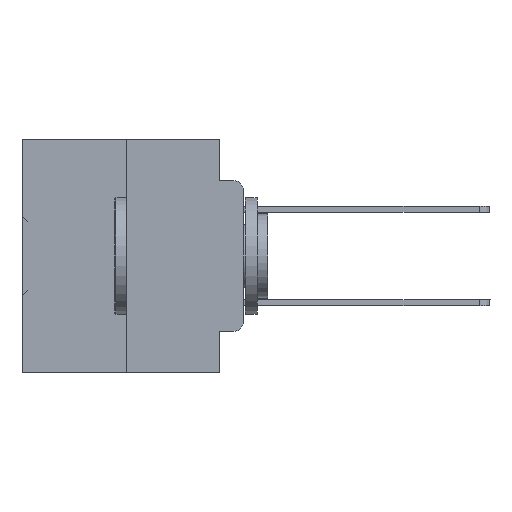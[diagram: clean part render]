
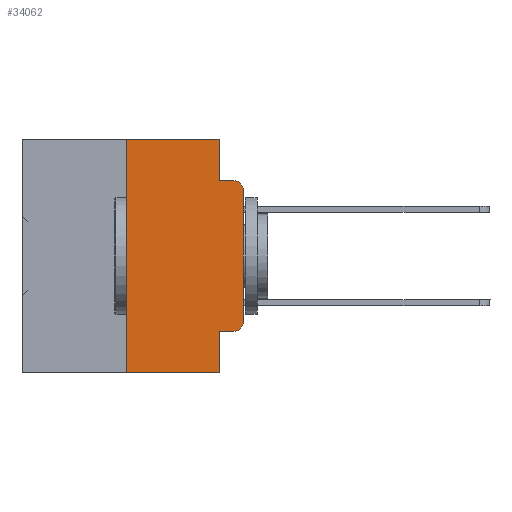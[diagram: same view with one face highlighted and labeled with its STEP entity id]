
A CAD part, left-side view. The second image highlights one B-rep face of the part: STEP entity #34062.
In plain terms, the highlighted planar face has unit normal (-1, 0, 0).
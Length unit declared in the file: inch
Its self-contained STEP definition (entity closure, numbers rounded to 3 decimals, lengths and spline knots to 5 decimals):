
#407 = VERTEX_POINT ( 'NONE', #38082 ) ;
#683 = VECTOR ( 'NONE', #4241, 39.37008 ) ;
#1294 = VERTEX_POINT ( 'NONE', #4804 ) ;
#1327 = CARTESIAN_POINT ( 'NONE',  ( 0., 0.02, -0.1085 ) ) ;
#2591 = VERTEX_POINT ( 'NONE', #18202 ) ;
#2975 = AXIS2_PLACEMENT_3D ( 'NONE', #17209, #35795, #11533 ) ;
#3467 = DIRECTION ( 'NONE',  ( 0., 0., 1. ) ) ;
#3710 = CARTESIAN_POINT ( 'NONE',  ( 0., 0.25, -0.5 ) ) ;
#3954 = VECTOR ( 'NONE', #31752, 39.37008 ) ;
#4241 = DIRECTION ( 'NONE',  ( 0., 0., 1. ) ) ;
#4332 = DIRECTION ( 'NONE',  ( 0., 0., -1. ) ) ;
#4364 = ORIENTED_EDGE ( 'NONE', *, *, #11351, .T. ) ;
#4804 = CARTESIAN_POINT ( 'NONE',  ( 0., 0.25, 0. ) ) ;
#6156 = DIRECTION ( 'NONE',  ( 0., -1., 0. ) ) ;
#6776 = DIRECTION ( 'NONE',  ( 0., 0., -1. ) ) ;
#6973 = DIRECTION ( 'NONE',  ( -1., 0., 0. ) ) ;
#7089 = VERTEX_POINT ( 'NONE', #38326 ) ;
#7437 = VERTEX_POINT ( 'NONE', #3710 ) ;
#8214 = VERTEX_POINT ( 'NONE', #8440 ) ;
#8440 = CARTESIAN_POINT ( 'NONE',  ( 0., 0.051, -0.5 ) ) ;
#8843 = VECTOR ( 'NONE', #4332, 39.37008 ) ;
#9955 = EDGE_CURVE ( 'NONE', #7089, #17361, #34268, .T. ) ;
#10130 = VERTEX_POINT ( 'NONE', #12639 ) ;
#11351 = EDGE_CURVE ( 'NONE', #17361, #12760, #29073, .T. ) ;
#11533 = DIRECTION ( 'NONE',  ( 0., 0., -1. ) ) ;
#11963 = EDGE_CURVE ( 'NONE', #2591, #26058, #12792, .T. ) ;
#12149 = CARTESIAN_POINT ( 'NONE',  ( 0., 0.25, 0. ) ) ;
#12639 = CARTESIAN_POINT ( 'NONE',  ( 0., 0.051, -0.4115 ) ) ;
#12760 = VERTEX_POINT ( 'NONE', #35801 ) ;
#12792 = LINE ( 'NONE', #28317, #3954 ) ;
#12915 = LINE ( 'NONE', #34125, #22692 ) ;
#13375 = LINE ( 'NONE', #31732, #28766 ) ;
#13603 = CIRCLE ( 'NONE', #23914, 0.02 ) ;
#14032 = LINE ( 'NONE', #31983, #8843 ) ;
#14511 = LINE ( 'NONE', #17930, #18230 ) ;
#15934 = EDGE_CURVE ( 'NONE', #7437, #1294, #37210, .T. ) ;
#17081 = EDGE_CURVE ( 'NONE', #12760, #26058, #13603, .T. ) ;
#17209 = CARTESIAN_POINT ( 'NONE',  ( 0., 0.473, 0. ) ) ;
#17314 = DIRECTION ( 'NONE',  ( 0., 0., -1. ) ) ;
#17361 = VERTEX_POINT ( 'NONE', #30176 ) ;
#17407 = VECTOR ( 'NONE', #3467, 39.37008 ) ;
#17795 = FACE_OUTER_BOUND ( 'NONE', #28862, .T. ) ;
#17930 = CARTESIAN_POINT ( 'NONE',  ( 0., 0.051, 0. ) ) ;
#18202 = CARTESIAN_POINT ( 'NONE',  ( 0., 0.051, -0.0885 ) ) ;
#18230 = VECTOR ( 'NONE', #26824, 39.37008 ) ;
#18238 = ORIENTED_EDGE ( 'NONE', *, *, #34760, .F. ) ;
#18348 = ORIENTED_EDGE ( 'NONE', *, *, #9955, .T. ) ;
#18713 = EDGE_CURVE ( 'NONE', #407, #2591, #14511, .T. ) ;
#19582 = EDGE_CURVE ( 'NONE', #1294, #407, #12915, .T. ) ;
#19588 = ORIENTED_EDGE ( 'NONE', *, *, #15934, .F. ) ;
#20094 = AXIS2_PLACEMENT_3D ( 'NONE', #33239, #32841, #17314 ) ;
#20213 = ORIENTED_EDGE ( 'NONE', *, *, #11963, .F. ) ;
#20420 = PLANE ( 'NONE',  #2975 ) ;
#21450 = VECTOR ( 'NONE', #6156, 39.37008 ) ;
#22692 = VECTOR ( 'NONE', #24830, 39.37008 ) ;
#23743 = LINE ( 'NONE', #36079, #21450 ) ;
#23748 = ORIENTED_EDGE ( 'NONE', *, *, #17081, .T. ) ;
#23914 = AXIS2_PLACEMENT_3D ( 'NONE', #1327, #6973, #6776 ) ;
#24830 = DIRECTION ( 'NONE',  ( 0., -1., 0. ) ) ;
#26058 = VERTEX_POINT ( 'NONE', #34453 ) ;
#26824 = DIRECTION ( 'NONE',  ( 0., 0., -1. ) ) ;
#27936 = ORIENTED_EDGE ( 'NONE', *, *, #18713, .F. ) ;
#28298 = DIRECTION ( 'NONE',  ( 0., -1., 0. ) ) ;
#28317 = CARTESIAN_POINT ( 'NONE',  ( 0., 0.051, -0.0885 ) ) ;
#28569 = ORIENTED_EDGE ( 'NONE', *, *, #28777, .T. ) ;
#28653 = ORIENTED_EDGE ( 'NONE', *, *, #19582, .F. ) ;
#28766 = VECTOR ( 'NONE', #28298, 39.37008 ) ;
#28777 = EDGE_CURVE ( 'NONE', #10130, #7089, #23743, .T. ) ;
#28862 = EDGE_LOOP ( 'NONE', ( #4364, #23748, #20213, #27936, #28653, #19588, #32619, #18238, #28569, #18348 ) ) ;
#29073 = LINE ( 'NONE', #35961, #683 ) ;
#30176 = CARTESIAN_POINT ( 'NONE',  ( 0., 0., -0.3915 ) ) ;
#31732 = CARTESIAN_POINT ( 'NONE',  ( 0., 0.473, -0.5 ) ) ;
#31752 = DIRECTION ( 'NONE',  ( 0., -1., 0. ) ) ;
#31983 = CARTESIAN_POINT ( 'NONE',  ( 0., 0.051, 0. ) ) ;
#32619 = ORIENTED_EDGE ( 'NONE', *, *, #33874, .T. ) ;
#32841 = DIRECTION ( 'NONE',  ( -1., 0., 0. ) ) ;
#33239 = CARTESIAN_POINT ( 'NONE',  ( 0., 0.02, -0.3915 ) ) ;
#33874 = EDGE_CURVE ( 'NONE', #7437, #8214, #13375, .T. ) ;
#34062 = ADVANCED_FACE ( 'NONE', ( #17795 ), #20420, .F. ) ;
#34125 = CARTESIAN_POINT ( 'NONE',  ( 0., 0.473, 0. ) ) ;
#34268 = CIRCLE ( 'NONE', #20094, 0.02 ) ;
#34453 = CARTESIAN_POINT ( 'NONE',  ( 0., 0.02, -0.0885 ) ) ;
#34760 = EDGE_CURVE ( 'NONE', #10130, #8214, #14032, .T. ) ;
#35795 = DIRECTION ( 'NONE',  ( 1., 0., 0. ) ) ;
#35801 = CARTESIAN_POINT ( 'NONE',  ( 0., 0., -0.1085 ) ) ;
#35961 = CARTESIAN_POINT ( 'NONE',  ( 0., 0., 0. ) ) ;
#36079 = CARTESIAN_POINT ( 'NONE',  ( 0., 0.051, -0.4115 ) ) ;
#37210 = LINE ( 'NONE', #12149, #17407 ) ;
#38082 = CARTESIAN_POINT ( 'NONE',  ( 0., 0.051, 0. ) ) ;
#38326 = CARTESIAN_POINT ( 'NONE',  ( 0., 0.02, -0.4115 ) ) ;
